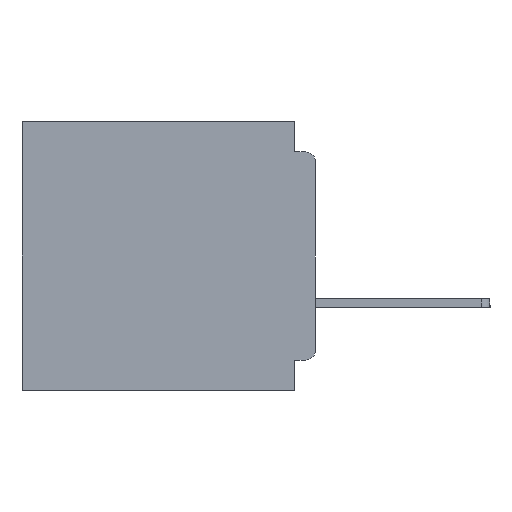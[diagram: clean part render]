
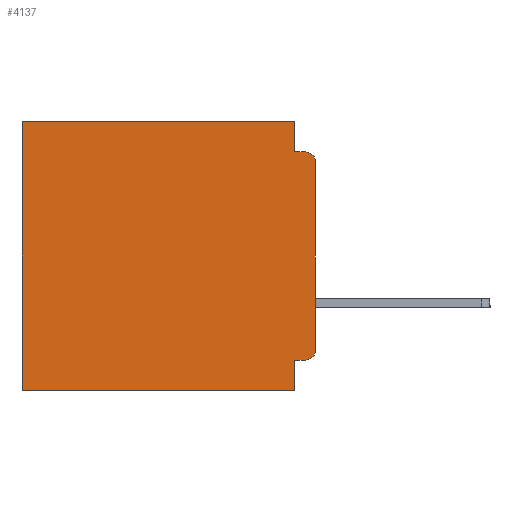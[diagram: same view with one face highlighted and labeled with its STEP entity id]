
A CAD part, left-side view. The second image highlights one B-rep face of the part: STEP entity #4137.
In plain terms, the highlighted planar face has unit normal (-1, 0, 0).
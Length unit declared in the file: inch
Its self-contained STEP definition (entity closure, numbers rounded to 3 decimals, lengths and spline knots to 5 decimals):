
#564 = CARTESIAN_POINT ( 'NONE',  ( 0.3, 0.437, -0.4 ) ) ;
#1112 = DIRECTION ( 'NONE',  ( 0., 1., 0. ) ) ;
#1616 = ORIENTED_EDGE ( 'NONE', *, *, #28156, .F. ) ;
#1880 = DIRECTION ( 'NONE',  ( 0., -1., 0. ) ) ;
#2324 = LINE ( 'NONE', #27184, #9663 ) ;
#2915 = VECTOR ( 'NONE', #1880, 39.37008 ) ;
#3504 = LINE ( 'NONE', #564, #18075 ) ;
#4137 = ADVANCED_FACE ( 'NONE', ( #16259 ), #18862, .F. ) ;
#4365 = ORIENTED_EDGE ( 'NONE', *, *, #22341, .F. ) ;
#4432 = DIRECTION ( 'NONE',  ( -1., 0., 0. ) ) ;
#4532 = EDGE_CURVE ( 'NONE', #19697, #6266, #11258, .T. ) ;
#4773 = AXIS2_PLACEMENT_3D ( 'NONE', #7135, #36363, #18988 ) ;
#5184 = CARTESIAN_POINT ( 'NONE',  ( 0.3, 0.437, -0.4 ) ) ;
#5925 = DIRECTION ( 'NONE',  ( -1., 0., 0. ) ) ;
#6196 = ORIENTED_EDGE ( 'NONE', *, *, #36927, .F. ) ;
#6266 = VERTEX_POINT ( 'NONE', #26345 ) ;
#6626 = ORIENTED_EDGE ( 'NONE', *, *, #21360, .T. ) ;
#7135 = CARTESIAN_POINT ( 'NONE',  ( 0.3, 0., -0.4 ) ) ;
#7325 = LINE ( 'NONE', #22528, #8229 ) ;
#7924 = EDGE_CURVE ( 'NONE', #21485, #25182, #2324, .T. ) ;
#7985 = DIRECTION ( 'NONE',  ( 0., 0., -1. ) ) ;
#8229 = VECTOR ( 'NONE', #7985, 39.37008 ) ;
#9663 = VECTOR ( 'NONE', #30112, 39.37008 ) ;
#9787 = CARTESIAN_POINT ( 'NONE',  ( 0.3, 0., -0.355 ) ) ;
#9835 = VECTOR ( 'NONE', #1112, 39.37008 ) ;
#10270 = ORIENTED_EDGE ( 'NONE', *, *, #19309, .T. ) ;
#10799 = VERTEX_POINT ( 'NONE', #34855 ) ;
#11023 = CARTESIAN_POINT ( 'NONE',  ( 0.3, 0.031, 0. ) ) ;
#11258 = LINE ( 'NONE', #32420, #31729 ) ;
#12266 = CARTESIAN_POINT ( 'NONE',  ( 0.3, 0.031, -0.4 ) ) ;
#14153 = CARTESIAN_POINT ( 'NONE',  ( 0.3, 0., -0.4 ) ) ;
#14308 = VERTEX_POINT ( 'NONE', #31805 ) ;
#14763 = EDGE_CURVE ( 'NONE', #14308, #25566, #26140, .T. ) ;
#15214 = VECTOR ( 'NONE', #17047, 39.37008 ) ;
#15400 = AXIS2_PLACEMENT_3D ( 'NONE', #21870, #4432, #24775 ) ;
#15486 = EDGE_CURVE ( 'NONE', #20100, #34126, #22896, .T. ) ;
#16259 = FACE_OUTER_BOUND ( 'NONE', #18159, .T. ) ;
#17040 = LINE ( 'NONE', #14153, #15214 ) ;
#17047 = DIRECTION ( 'NONE',  ( 0., 0., -1. ) ) ;
#17079 = ORIENTED_EDGE ( 'NONE', *, *, #4532, .T. ) ;
#17808 = CARTESIAN_POINT ( 'NONE',  ( 0.3, 0., -0.34 ) ) ;
#17923 = DIRECTION ( 'NONE',  ( 0., 1., 0. ) ) ;
#18075 = VECTOR ( 'NONE', #23876, 39.37008 ) ;
#18159 = EDGE_LOOP ( 'NONE', ( #21187, #6626, #30752, #1616, #17079, #10270, #26669, #4365, #6196, #29408 ) ) ;
#18488 = LINE ( 'NONE', #9787, #9835 ) ;
#18862 = PLANE ( 'NONE',  #4773 ) ;
#18988 = DIRECTION ( 'NONE',  ( 0., 0., -1. ) ) ;
#19309 = EDGE_CURVE ( 'NONE', #6266, #25182, #3504, .T. ) ;
#19697 = VERTEX_POINT ( 'NONE', #11023 ) ;
#20100 = VERTEX_POINT ( 'NONE', #24588 ) ;
#20497 = DIRECTION ( 'NONE',  ( 0., 0., -1. ) ) ;
#21187 = ORIENTED_EDGE ( 'NONE', *, *, #30377, .F. ) ;
#21360 = EDGE_CURVE ( 'NONE', #10799, #25566, #33332, .T. ) ;
#21485 = VERTEX_POINT ( 'NONE', #12266 ) ;
#21870 = CARTESIAN_POINT ( 'NONE',  ( 0.3, 0.015, -0.34 ) ) ;
#22341 = EDGE_CURVE ( 'NONE', #26843, #21485, #7325, .T. ) ;
#22528 = CARTESIAN_POINT ( 'NONE',  ( 0.3, 0.031, -0.4 ) ) ;
#22896 = CIRCLE ( 'NONE', #15400, 0.015 ) ;
#23340 = CARTESIAN_POINT ( 'NONE',  ( 0.3, 0.015, -0.06 ) ) ;
#23876 = DIRECTION ( 'NONE',  ( 0., 0., -1. ) ) ;
#24588 = CARTESIAN_POINT ( 'NONE',  ( 0.3, 0.015, -0.355 ) ) ;
#24775 = DIRECTION ( 'NONE',  ( 0., 0., -1. ) ) ;
#25182 = VERTEX_POINT ( 'NONE', #5184 ) ;
#25566 = VERTEX_POINT ( 'NONE', #32979 ) ;
#26140 = LINE ( 'NONE', #33916, #2915 ) ;
#26255 = DIRECTION ( 'NONE',  ( 0., 0., -1. ) ) ;
#26345 = CARTESIAN_POINT ( 'NONE',  ( 0.3, 0.437, 0. ) ) ;
#26669 = ORIENTED_EDGE ( 'NONE', *, *, #7924, .F. ) ;
#26843 = VERTEX_POINT ( 'NONE', #34689 ) ;
#27184 = CARTESIAN_POINT ( 'NONE',  ( 0.3, 0., -0.4 ) ) ;
#28156 = EDGE_CURVE ( 'NONE', #19697, #14308, #34529, .T. ) ;
#29408 = ORIENTED_EDGE ( 'NONE', *, *, #15486, .T. ) ;
#30112 = DIRECTION ( 'NONE',  ( 0., 1., 0. ) ) ;
#30377 = EDGE_CURVE ( 'NONE', #10799, #34126, #17040, .T. ) ;
#30752 = ORIENTED_EDGE ( 'NONE', *, *, #14763, .F. ) ;
#31729 = VECTOR ( 'NONE', #17923, 39.37008 ) ;
#31805 = CARTESIAN_POINT ( 'NONE',  ( 0.3, 0.031, -0.045 ) ) ;
#32062 = CARTESIAN_POINT ( 'NONE',  ( 0.3, 0.031, 0. ) ) ;
#32420 = CARTESIAN_POINT ( 'NONE',  ( 0.3, 0., 0. ) ) ;
#32979 = CARTESIAN_POINT ( 'NONE',  ( 0.3, 0.015, -0.045 ) ) ;
#33332 = CIRCLE ( 'NONE', #36500, 0.015 ) ;
#33620 = VECTOR ( 'NONE', #20497, 39.37008 ) ;
#33916 = CARTESIAN_POINT ( 'NONE',  ( 0.3, 0., -0.045 ) ) ;
#34126 = VERTEX_POINT ( 'NONE', #17808 ) ;
#34529 = LINE ( 'NONE', #32062, #33620 ) ;
#34689 = CARTESIAN_POINT ( 'NONE',  ( 0.3, 0.031, -0.355 ) ) ;
#34855 = CARTESIAN_POINT ( 'NONE',  ( 0.3, 0., -0.06 ) ) ;
#36363 = DIRECTION ( 'NONE',  ( 1., 0., 0. ) ) ;
#36500 = AXIS2_PLACEMENT_3D ( 'NONE', #23340, #5925, #26255 ) ;
#36927 = EDGE_CURVE ( 'NONE', #20100, #26843, #18488, .T. ) ;
